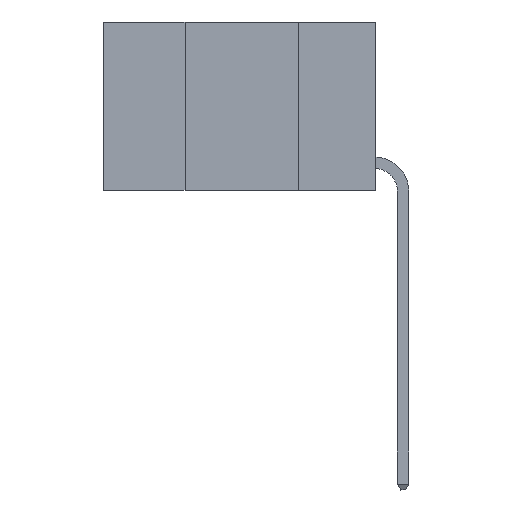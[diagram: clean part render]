
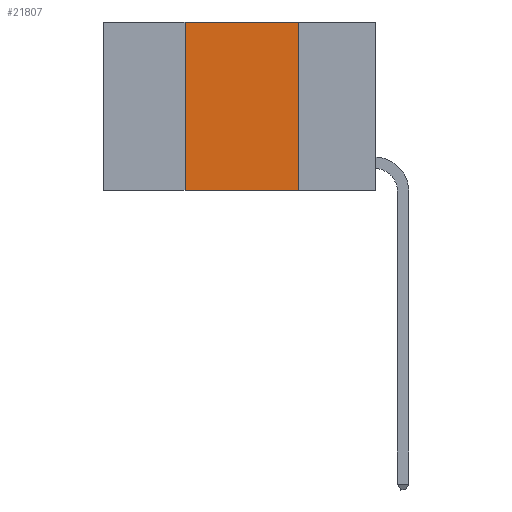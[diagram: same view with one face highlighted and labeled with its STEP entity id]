
A CAD part, left-side view. The second image highlights one B-rep face of the part: STEP entity #21807.
In plain terms, the highlighted planar face has unit normal (-1, 0, 0).
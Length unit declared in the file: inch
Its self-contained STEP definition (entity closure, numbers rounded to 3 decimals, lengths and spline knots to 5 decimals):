
#298 = EDGE_CURVE ( 'NONE', #25267, #15955, #22659, .T. ) ;
#1951 = LINE ( 'NONE', #8251, #16325 ) ;
#3226 = LINE ( 'NONE', #9096, #26363 ) ;
#3315 = ORIENTED_EDGE ( 'NONE', *, *, #3521, .F. ) ;
#3455 = CARTESIAN_POINT ( 'NONE',  ( 0., 0.17, 0. ) ) ;
#3521 = EDGE_CURVE ( 'NONE', #25899, #18418, #1951, .T. ) ;
#5380 = CARTESIAN_POINT ( 'NONE',  ( 0., 0.17, 0. ) ) ;
#5977 = DIRECTION ( 'NONE',  ( 1., 0., 0. ) ) ;
#6087 = ORIENTED_EDGE ( 'NONE', *, *, #26111, .T. ) ;
#6108 = DIRECTION ( 'NONE',  ( 0., 0., -1. ) ) ;
#6263 = CARTESIAN_POINT ( 'NONE',  ( 0., 0.6, 0. ) ) ;
#6388 = PLANE ( 'NONE',  #13177 ) ;
#8251 = CARTESIAN_POINT ( 'NONE',  ( 0., 0.42, 0. ) ) ;
#9096 = CARTESIAN_POINT ( 'NONE',  ( 0., 0.6, -0.37 ) ) ;
#10800 = CARTESIAN_POINT ( 'NONE',  ( 0., 0.42, -0.37 ) ) ;
#10802 = EDGE_CURVE ( 'NONE', #18418, #25267, #14644, .T. ) ;
#11601 = CARTESIAN_POINT ( 'NONE',  ( 0., 0.42, 0. ) ) ;
#12685 = VECTOR ( 'NONE', #20562, 39.37008 ) ;
#12704 = DIRECTION ( 'NONE',  ( 0., -1., 0. ) ) ;
#13177 = AXIS2_PLACEMENT_3D ( 'NONE', #16877, #5977, #6108 ) ;
#14644 = LINE ( 'NONE', #6263, #16853 ) ;
#14769 = FACE_OUTER_BOUND ( 'NONE', #26362, .T. ) ;
#15955 = VERTEX_POINT ( 'NONE', #25444 ) ;
#16325 = VECTOR ( 'NONE', #20766, 39.37008 ) ;
#16853 = VECTOR ( 'NONE', #12704, 39.37008 ) ;
#16877 = CARTESIAN_POINT ( 'NONE',  ( 0., 0.6, 0. ) ) ;
#18418 = VERTEX_POINT ( 'NONE', #11601 ) ;
#20562 = DIRECTION ( 'NONE',  ( 0., 0., -1. ) ) ;
#20766 = DIRECTION ( 'NONE',  ( 0., 0., 1. ) ) ;
#21807 = ADVANCED_FACE ( 'NONE', ( #14769 ), #6388, .F. ) ;
#22659 = LINE ( 'NONE', #3455, #12685 ) ;
#25267 = VERTEX_POINT ( 'NONE', #5380 ) ;
#25444 = CARTESIAN_POINT ( 'NONE',  ( 0., 0.17, -0.37 ) ) ;
#25562 = ORIENTED_EDGE ( 'NONE', *, *, #10802, .F. ) ;
#25899 = VERTEX_POINT ( 'NONE', #10800 ) ;
#26111 = EDGE_CURVE ( 'NONE', #25899, #15955, #3226, .T. ) ;
#26228 = DIRECTION ( 'NONE',  ( 0., -1., 0. ) ) ;
#26362 = EDGE_LOOP ( 'NONE', ( #27633, #25562, #3315, #6087 ) ) ;
#26363 = VECTOR ( 'NONE', #26228, 39.37008 ) ;
#27633 = ORIENTED_EDGE ( 'NONE', *, *, #298, .F. ) ;
